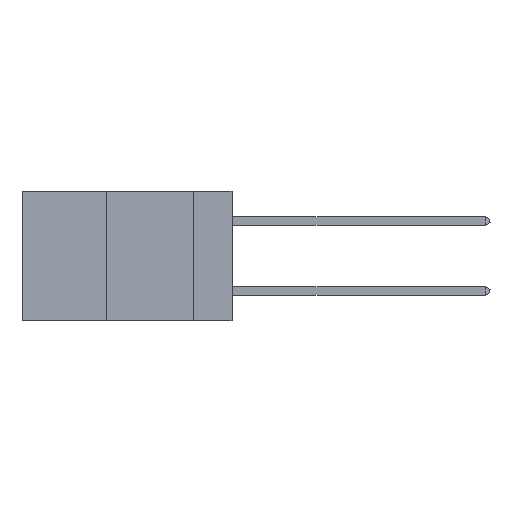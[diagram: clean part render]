
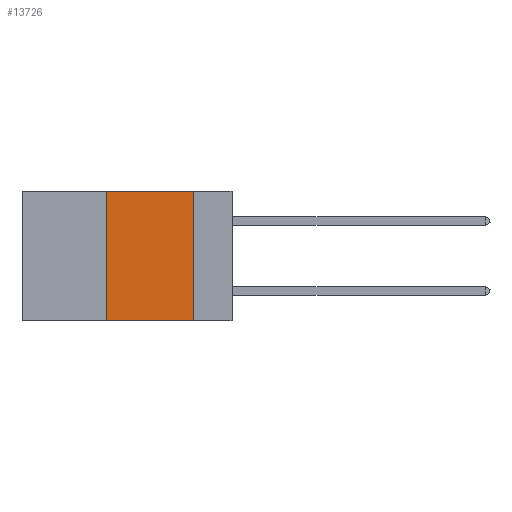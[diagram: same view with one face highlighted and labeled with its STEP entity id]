
A CAD part, left-side view. The second image highlights one B-rep face of the part: STEP entity #13726.
In plain terms, the highlighted planar face has unit normal (-1, 0, 0).
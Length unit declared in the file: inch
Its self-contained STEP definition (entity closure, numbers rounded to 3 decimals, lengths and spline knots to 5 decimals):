
#797 = LINE ( 'NONE', #21817, #19629 ) ;
#2131 = VERTEX_POINT ( 'NONE', #8950 ) ;
#2317 = EDGE_CURVE ( 'NONE', #28050, #4770, #11026, .T. ) ;
#2342 = CARTESIAN_POINT ( 'NONE',  ( 0., 0.11, 0. ) ) ;
#3371 = FACE_OUTER_BOUND ( 'NONE', #23229, .T. ) ;
#3630 = VECTOR ( 'NONE', #28859, 39.37008 ) ;
#3796 = DIRECTION ( 'NONE',  ( 0., -1., 0. ) ) ;
#4492 = VECTOR ( 'NONE', #7062, 39.37008 ) ;
#4557 = EDGE_CURVE ( 'NONE', #2131, #15746, #797, .T. ) ;
#4764 = LINE ( 'NONE', #14034, #3630 ) ;
#4770 = VERTEX_POINT ( 'NONE', #17737 ) ;
#4897 = DIRECTION ( 'NONE',  ( 0., 0., 1. ) ) ;
#6994 = ORIENTED_EDGE ( 'NONE', *, *, #24919, .T. ) ;
#7062 = DIRECTION ( 'NONE',  ( 0., 0., -1. ) ) ;
#8397 = EDGE_CURVE ( 'NONE', #15746, #28050, #4764, .T. ) ;
#8912 = ORIENTED_EDGE ( 'NONE', *, *, #2317, .F. ) ;
#8950 = CARTESIAN_POINT ( 'NONE',  ( 0., 0.36, -0.37 ) ) ;
#9730 = VECTOR ( 'NONE', #3796, 39.37008 ) ;
#11026 = LINE ( 'NONE', #2342, #4492 ) ;
#11634 = LINE ( 'NONE', #23607, #9730 ) ;
#11926 = ORIENTED_EDGE ( 'NONE', *, *, #8397, .F. ) ;
#12538 = CARTESIAN_POINT ( 'NONE',  ( 0., 0.11, 0. ) ) ;
#13726 = ADVANCED_FACE ( 'NONE', ( #3371 ), #30513, .F. ) ;
#14034 = CARTESIAN_POINT ( 'NONE',  ( 0., 0.6, 0. ) ) ;
#15144 = ORIENTED_EDGE ( 'NONE', *, *, #4557, .F. ) ;
#15746 = VERTEX_POINT ( 'NONE', #18518 ) ;
#17737 = CARTESIAN_POINT ( 'NONE',  ( 0., 0.11, -0.37 ) ) ;
#18518 = CARTESIAN_POINT ( 'NONE',  ( 0., 0.36, 0. ) ) ;
#19629 = VECTOR ( 'NONE', #4897, 39.37008 ) ;
#20550 = AXIS2_PLACEMENT_3D ( 'NONE', #25658, #20758, #30619 ) ;
#20758 = DIRECTION ( 'NONE',  ( 1., 0., 0. ) ) ;
#21817 = CARTESIAN_POINT ( 'NONE',  ( 0., 0.36, 0. ) ) ;
#23229 = EDGE_LOOP ( 'NONE', ( #8912, #11926, #15144, #6994 ) ) ;
#23607 = CARTESIAN_POINT ( 'NONE',  ( 0., 0.6, -0.37 ) ) ;
#24919 = EDGE_CURVE ( 'NONE', #2131, #4770, #11634, .T. ) ;
#25658 = CARTESIAN_POINT ( 'NONE',  ( 0., 0.6, 0. ) ) ;
#28050 = VERTEX_POINT ( 'NONE', #12538 ) ;
#28859 = DIRECTION ( 'NONE',  ( 0., -1., 0. ) ) ;
#30513 = PLANE ( 'NONE',  #20550 ) ;
#30619 = DIRECTION ( 'NONE',  ( 0., 0., -1. ) ) ;
